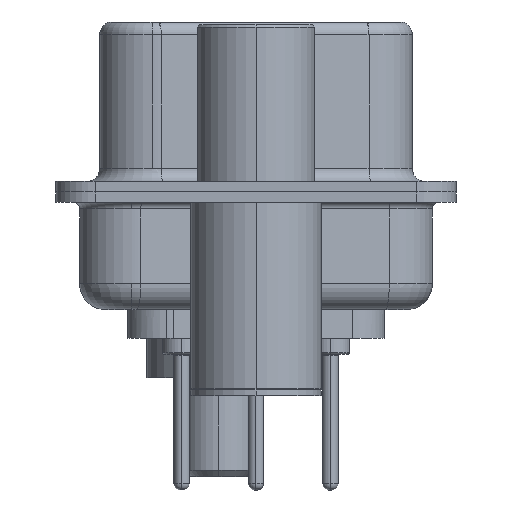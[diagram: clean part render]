
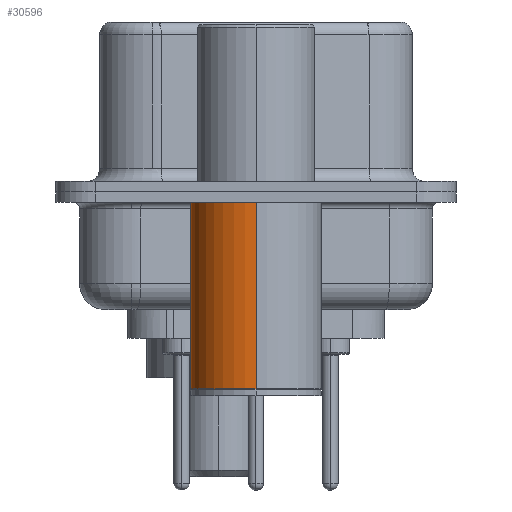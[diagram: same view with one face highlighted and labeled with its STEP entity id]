
A CAD part, left-side view. The second image highlights one B-rep face of the part: STEP entity #30596.
In plain terms, the highlighted cylindrical face has radius 2.5 mm (diameter 5 mm), a partial arc.
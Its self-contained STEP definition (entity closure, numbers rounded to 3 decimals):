
#42 = CARTESIAN_POINT ( 'NONE',  ( 0., 0., -0.4 ) ) ;
#504 = VECTOR ( 'NONE', #8440, 1000. ) ;
#532 = LINE ( 'NONE', #9889, #22280 ) ;
#2864 = DIRECTION ( 'NONE',  ( 1., 0., 0. ) ) ;
#3266 = EDGE_CURVE ( 'NONE', #31283, #24718, #532, .T. ) ;
#4005 = LINE ( 'NONE', #27232, #504 ) ;
#7773 = DIRECTION ( 'NONE',  ( 0., 0., 1. ) ) ;
#8440 = DIRECTION ( 'NONE',  ( 0., 0., 1. ) ) ;
#8715 = EDGE_CURVE ( 'NONE', #23731, #31283, #34364, .T. ) ;
#9524 = AXIS2_PLACEMENT_3D ( 'NONE', #17229, #22776, #25502 ) ;
#9889 = CARTESIAN_POINT ( 'NONE',  ( -2.5, 0., 0.581 ) ) ;
#10070 = CARTESIAN_POINT ( 'NONE',  ( 2.5, 0., -7.525 ) ) ;
#10173 = ORIENTED_EDGE ( 'NONE', *, *, #13081, .F. ) ;
#11112 = CIRCLE ( 'NONE', #28062, 2.5 ) ;
#13081 = EDGE_CURVE ( 'NONE', #15271, #24718, #11112, .T. ) ;
#15271 = VERTEX_POINT ( 'NONE', #15994 ) ;
#15994 = CARTESIAN_POINT ( 'NONE',  ( 2.5, 0., -0.4 ) ) ;
#17229 = CARTESIAN_POINT ( 'NONE',  ( 0., 0., 0.581 ) ) ;
#17233 = CYLINDRICAL_SURFACE ( 'NONE', #9524, 2.5 ) ;
#17756 = EDGE_LOOP ( 'NONE', ( #20650, #21826, #10173, #21601 ) ) ;
#18105 = FACE_OUTER_BOUND ( 'NONE', #17756, .T. ) ;
#19153 = DIRECTION ( 'NONE',  ( 0., 0., 1. ) ) ;
#20650 = ORIENTED_EDGE ( 'NONE', *, *, #8715, .T. ) ;
#20695 = DIRECTION ( 'NONE',  ( 0., 0., 1. ) ) ;
#21601 = ORIENTED_EDGE ( 'NONE', *, *, #32015, .F. ) ;
#21826 = ORIENTED_EDGE ( 'NONE', *, *, #3266, .T. ) ;
#22280 = VECTOR ( 'NONE', #20695, 1000. ) ;
#22654 = CARTESIAN_POINT ( 'NONE',  ( -2.5, 0., -0.4 ) ) ;
#22776 = DIRECTION ( 'NONE',  ( 0., 0., 1. ) ) ;
#22888 = CARTESIAN_POINT ( 'NONE',  ( -2.5, 0., -7.525 ) ) ;
#23731 = VERTEX_POINT ( 'NONE', #10070 ) ;
#23953 = CARTESIAN_POINT ( 'NONE',  ( 0., 0., -7.525 ) ) ;
#24718 = VERTEX_POINT ( 'NONE', #22654 ) ;
#25502 = DIRECTION ( 'NONE',  ( 1., 0., 0. ) ) ;
#26685 = DIRECTION ( 'NONE',  ( 1., 0., 0. ) ) ;
#27232 = CARTESIAN_POINT ( 'NONE',  ( 2.5, 0., 0.581 ) ) ;
#28062 = AXIS2_PLACEMENT_3D ( 'NONE', #42, #19153, #2864 ) ;
#30596 = ADVANCED_FACE ( 'NONE', ( #18105 ), #17233, .T. ) ;
#31283 = VERTEX_POINT ( 'NONE', #22888 ) ;
#32015 = EDGE_CURVE ( 'NONE', #23731, #15271, #4005, .T. ) ;
#32288 = AXIS2_PLACEMENT_3D ( 'NONE', #23953, #7773, #26685 ) ;
#34364 = CIRCLE ( 'NONE', #32288, 2.5 ) ;
